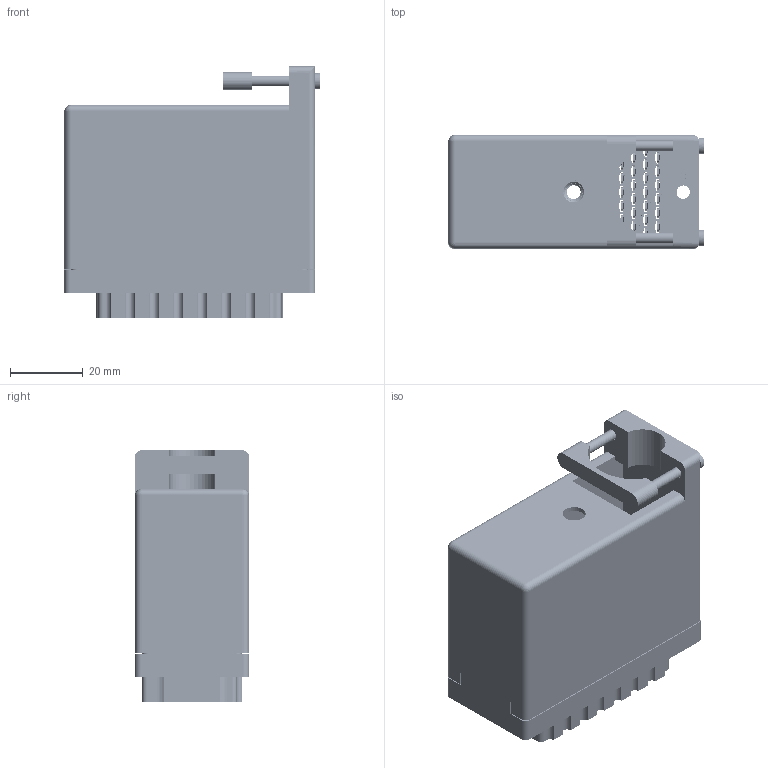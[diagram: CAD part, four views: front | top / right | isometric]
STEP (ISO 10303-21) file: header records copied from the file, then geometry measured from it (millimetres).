
FILE_DESCRIPTION (( 'STEP AP203' ), '1' );
FILE_NAME ('516-090-501-666.STEP', '2020-09-08T18:42:08', ( '' ), ( '' ), 'SwSTEP 2.0', 'SolidWorks 2020', '' );
FILE_SCHEMA (( 'CONFIG_CONTROL_DESIGN' ));
Length unit declared in the file: inch
Products named in the file (5): 516-292-001_501 Contact; 516-252-095-100; 516-090-501-666; 516-230-001_Metal - 090 Top Entry; 516 Part Receptacle_090
Assembly tree (94 placements, depth 2):
  516-090-501-666
    516 Part Receptacle_090
    516-292-001_501 Contact  x91
    516-230-001_Metal - 090 Top Entry
    516-252-095-100
Bounding box: 70.31 x 31.34 x 69.24 mm (x, y, z)
Volume: 38902.7 mm3; surface area: 69230.9 mm2
Topology: 94 solids, 94 shells, 8590 faces, 24951 edges, 16565 vertices
Faces by surface type: plane 5150, cylinder 2874, bspline 552, cone 12, sphere 2
Entity records: 76322 total; most frequent: CARTESIAN_POINT 14908, ORIENTED_EDGE 12458, DIRECTION 12122, EDGE_CURVE 6229, LINE 4550, VECTOR 4550, VERTEX_POINT 4145, AXIS2_PLACEMENT_3D 3786
